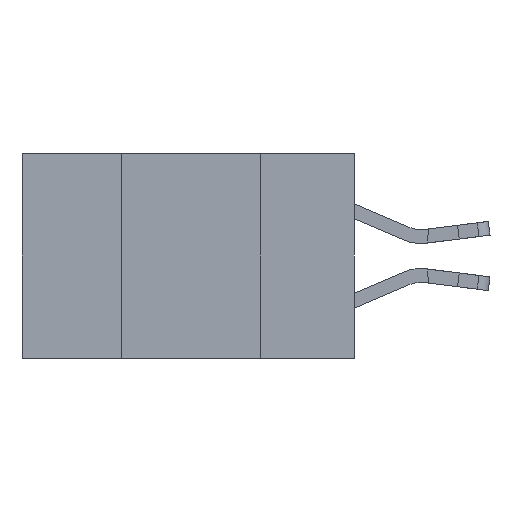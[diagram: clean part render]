
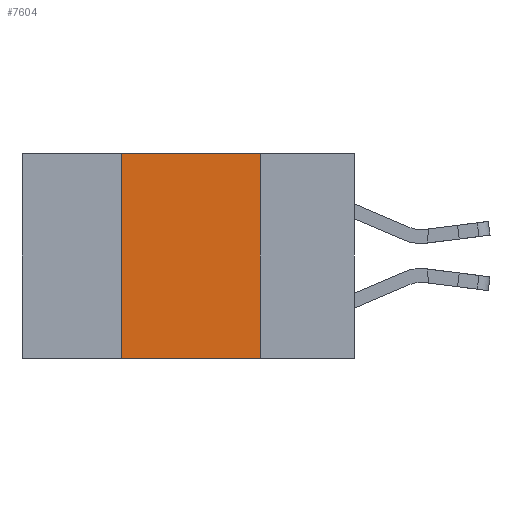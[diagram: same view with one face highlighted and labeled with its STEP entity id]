
A CAD part, left-side view. The second image highlights one B-rep face of the part: STEP entity #7604.
In plain terms, the highlighted planar face has unit normal (-1, 0, 0).
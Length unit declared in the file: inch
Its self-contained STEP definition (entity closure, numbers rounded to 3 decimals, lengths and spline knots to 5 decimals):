
#17 = EDGE_CURVE ( 'NONE', #19741, #13897, #14706, .T. ) ;
#735 = CARTESIAN_POINT ( 'NONE',  ( 0., 0.17, 0. ) ) ;
#1867 = FACE_OUTER_BOUND ( 'NONE', #16462, .T. ) ;
#2504 = DIRECTION ( 'NONE',  ( 1., 0., 0. ) ) ;
#4384 = LINE ( 'NONE', #8472, #20468 ) ;
#5656 = ORIENTED_EDGE ( 'NONE', *, *, #21632, .T. ) ;
#5750 = VERTEX_POINT ( 'NONE', #735 ) ;
#6374 = DIRECTION ( 'NONE',  ( 0., 0., -1. ) ) ;
#6941 = DIRECTION ( 'NONE',  ( 0., -1., 0. ) ) ;
#7054 = LINE ( 'NONE', #17496, #23118 ) ;
#7373 = CARTESIAN_POINT ( 'NONE',  ( 0., 0.42, 0. ) ) ;
#7579 = ORIENTED_EDGE ( 'NONE', *, *, #18739, .F. ) ;
#7604 = ADVANCED_FACE ( 'NONE', ( #1867 ), #15103, .F. ) ;
#8472 = CARTESIAN_POINT ( 'NONE',  ( 0., 0.17, 0. ) ) ;
#8733 = CARTESIAN_POINT ( 'NONE',  ( 0., 0.6, 0. ) ) ;
#12787 = CARTESIAN_POINT ( 'NONE',  ( 0., 0.42, -0.37 ) ) ;
#13844 = ORIENTED_EDGE ( 'NONE', *, *, #19708, .F. ) ;
#13897 = VERTEX_POINT ( 'NONE', #25852 ) ;
#14125 = VECTOR ( 'NONE', #16477, 39.37008 ) ;
#14706 = LINE ( 'NONE', #7373, #20919 ) ;
#15103 = PLANE ( 'NONE',  #19803 ) ;
#16061 = DIRECTION ( 'NONE',  ( 0., 0., 1. ) ) ;
#16462 = EDGE_LOOP ( 'NONE', ( #13844, #7579, #22693, #5656 ) ) ;
#16477 = DIRECTION ( 'NONE',  ( 0., -1., 0. ) ) ;
#17204 = DIRECTION ( 'NONE',  ( 0., 0., -1. ) ) ;
#17496 = CARTESIAN_POINT ( 'NONE',  ( 0., 0.6, 0. ) ) ;
#18217 = VERTEX_POINT ( 'NONE', #19988 ) ;
#18567 = CARTESIAN_POINT ( 'NONE',  ( 0., 0.6, -0.37 ) ) ;
#18739 = EDGE_CURVE ( 'NONE', #13897, #5750, #7054, .T. ) ;
#19708 = EDGE_CURVE ( 'NONE', #5750, #18217, #4384, .T. ) ;
#19741 = VERTEX_POINT ( 'NONE', #12787 ) ;
#19803 = AXIS2_PLACEMENT_3D ( 'NONE', #8733, #2504, #17204 ) ;
#19988 = CARTESIAN_POINT ( 'NONE',  ( 0., 0.17, -0.37 ) ) ;
#20348 = LINE ( 'NONE', #18567, #14125 ) ;
#20468 = VECTOR ( 'NONE', #6374, 39.37008 ) ;
#20919 = VECTOR ( 'NONE', #16061, 39.37008 ) ;
#21632 = EDGE_CURVE ( 'NONE', #19741, #18217, #20348, .T. ) ;
#22693 = ORIENTED_EDGE ( 'NONE', *, *, #17, .F. ) ;
#23118 = VECTOR ( 'NONE', #6941, 39.37008 ) ;
#25852 = CARTESIAN_POINT ( 'NONE',  ( 0., 0.42, 0. ) ) ;
